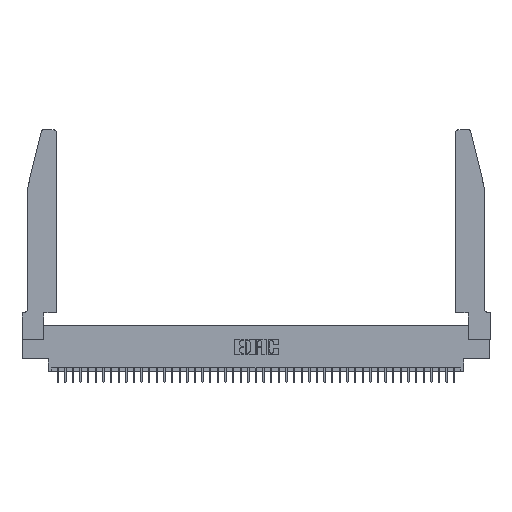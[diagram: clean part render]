
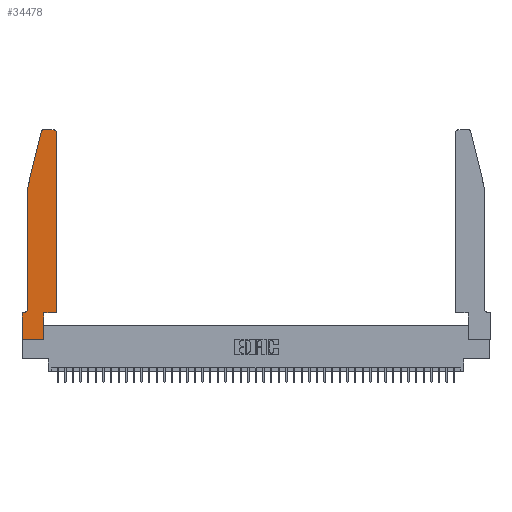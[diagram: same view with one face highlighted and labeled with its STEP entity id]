
A CAD part, top view. The second image highlights one B-rep face of the part: STEP entity #34478.
In plain terms, the highlighted planar face has unit normal (0, 0, 1).
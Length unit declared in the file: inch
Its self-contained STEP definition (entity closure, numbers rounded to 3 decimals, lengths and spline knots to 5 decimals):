
#2469 = ORIENTED_EDGE ( 'NONE', *, *, #20952, .T. ) ;
#2894 = VERTEX_POINT ( 'NONE', #5414 ) ;
#3393 = LINE ( 'NONE', #13477, #7256 ) ;
#3752 = VECTOR ( 'NONE', #13793, 39.37008 ) ;
#3867 = DIRECTION ( 'NONE',  ( -1., 0., 0. ) ) ;
#4237 = ORIENTED_EDGE ( 'NONE', *, *, #17763, .T. ) ;
#4721 = VERTEX_POINT ( 'NONE', #37767 ) ;
#4856 = VERTEX_POINT ( 'NONE', #15403 ) ;
#5414 = CARTESIAN_POINT ( 'NONE',  ( 0.4205, 2.75, 0.37 ) ) ;
#6735 = DIRECTION ( 'NONE',  ( -0.239, -0.971, 0. ) ) ;
#6791 = DIRECTION ( 'NONE',  ( 0., 0., -1. ) ) ;
#6862 = CIRCLE ( 'NONE', #9811, 0.07 ) ;
#7106 = CARTESIAN_POINT ( 'NONE',  ( 0., 0.35, 0.37 ) ) ;
#7256 = VECTOR ( 'NONE', #27380, 39.37008 ) ;
#7772 = ORIENTED_EDGE ( 'NONE', *, *, #38119, .T. ) ;
#7897 = CARTESIAN_POINT ( 'NONE',  ( 0.2865, 0., 0.37 ) ) ;
#8594 = VERTEX_POINT ( 'NONE', #33508 ) ;
#8915 = VERTEX_POINT ( 'NONE', #7897 ) ;
#9157 = ORIENTED_EDGE ( 'NONE', *, *, #35785, .T. ) ;
#9811 = AXIS2_PLACEMENT_3D ( 'NONE', #41248, #6791, #37839 ) ;
#9848 = ORIENTED_EDGE ( 'NONE', *, *, #42678, .T. ) ;
#10182 = ORIENTED_EDGE ( 'NONE', *, *, #14208, .T. ) ;
#10358 = CARTESIAN_POINT ( 'NONE',  ( 0.4505, 0.35, 0.37 ) ) ;
#10992 = VECTOR ( 'NONE', #33091, 39.37008 ) ;
#11718 = EDGE_CURVE ( 'NONE', #22660, #11918, #16778, .T. ) ;
#11918 = VERTEX_POINT ( 'NONE', #24294 ) ;
#13005 = ORIENTED_EDGE ( 'NONE', *, *, #24244, .T. ) ;
#13048 = DIRECTION ( 'NONE',  ( 0., -1., 0. ) ) ;
#13164 = DIRECTION ( 'NONE',  ( 0., 0., 1. ) ) ;
#13477 = CARTESIAN_POINT ( 'NONE',  ( 0., 0., 0.37 ) ) ;
#13793 = DIRECTION ( 'NONE',  ( 0., 1., 0. ) ) ;
#14169 = CARTESIAN_POINT ( 'NONE',  ( 0.2605, 2.75, 0.37 ) ) ;
#14208 = EDGE_CURVE ( 'NONE', #8915, #22660, #39485, .T. ) ;
#14546 = CARTESIAN_POINT ( 'NONE',  ( 0.2865, 0.35, 0.37 ) ) ;
#14649 = FACE_OUTER_BOUND ( 'NONE', #22229, .T. ) ;
#14872 = DIRECTION ( 'NONE',  ( 1., 0., 0. ) ) ;
#15403 = CARTESIAN_POINT ( 'NONE',  ( 0.0755, 0.42, 0.37 ) ) ;
#15844 = AXIS2_PLACEMENT_3D ( 'NONE', #7106, #38838, #14872 ) ;
#16377 = CARTESIAN_POINT ( 'NONE',  ( 0.4205, 2.72, 0.37 ) ) ;
#16703 = LINE ( 'NONE', #20130, #23182 ) ;
#16778 = LINE ( 'NONE', #33859, #42130 ) ;
#16821 = LINE ( 'NONE', #20233, #24595 ) ;
#17763 = EDGE_CURVE ( 'NONE', #8594, #4721, #25350, .T. ) ;
#17779 = EDGE_CURVE ( 'NONE', #2894, #39701, #24451, .T. ) ;
#18990 = CARTESIAN_POINT ( 'NONE',  ( 0.2865, 0.35, 0.37 ) ) ;
#19395 = CARTESIAN_POINT ( 'NONE',  ( 0.0755, 2., 0.37 ) ) ;
#20130 = CARTESIAN_POINT ( 'NONE',  ( 0.0755, 2., 0.37 ) ) ;
#20233 = CARTESIAN_POINT ( 'NONE',  ( 0.0755, 2., 0.37 ) ) ;
#20424 = LINE ( 'NONE', #38190, #29320 ) ;
#20952 = EDGE_CURVE ( 'NONE', #39519, #2894, #44147, .T. ) ;
#22229 = EDGE_LOOP ( 'NONE', ( #31428, #36930, #13005, #9157, #42473, #4237, #7772, #30737, #10182, #41584, #9848, #2469 ) ) ;
#22246 = CARTESIAN_POINT ( 'NONE',  ( 0., 0., 0.37 ) ) ;
#22268 = VECTOR ( 'NONE', #28747, 39.37008 ) ;
#22387 = VERTEX_POINT ( 'NONE', #19395 ) ;
#22660 = VERTEX_POINT ( 'NONE', #14546 ) ;
#23182 = VECTOR ( 'NONE', #13048, 39.37008 ) ;
#24244 = EDGE_CURVE ( 'NONE', #29957, #22387, #16821, .T. ) ;
#24294 = CARTESIAN_POINT ( 'NONE',  ( 0.4505, 0.35, 0.37 ) ) ;
#24451 = LINE ( 'NONE', #14169, #25905 ) ;
#24595 = VECTOR ( 'NONE', #6735, 39.37008 ) ;
#25350 = LINE ( 'NONE', #34931, #22268 ) ;
#25905 = VECTOR ( 'NONE', #3867, 39.37008 ) ;
#25978 = AXIS2_PLACEMENT_3D ( 'NONE', #16377, #40538, #34155 ) ;
#26748 = CARTESIAN_POINT ( 'NONE',  ( 0.25487, 2.72718, 0.37 ) ) ;
#27070 = DIRECTION ( 'NONE',  ( 1., 0., 0. ) ) ;
#27380 = DIRECTION ( 'NONE',  ( 0., -1., 0. ) ) ;
#28747 = DIRECTION ( 'NONE',  ( -1., 0., 0. ) ) ;
#29320 = VECTOR ( 'NONE', #37507, 39.37008 ) ;
#29957 = VERTEX_POINT ( 'NONE', #26748 ) ;
#30478 = CARTESIAN_POINT ( 'NONE',  ( 0.284, 2.72, 0.37 ) ) ;
#30737 = ORIENTED_EDGE ( 'NONE', *, *, #42673, .T. ) ;
#31428 = ORIENTED_EDGE ( 'NONE', *, *, #17779, .T. ) ;
#31615 = EDGE_CURVE ( 'NONE', #4856, #8594, #6862, .T. ) ;
#32009 = AXIS2_PLACEMENT_3D ( 'NONE', #30478, #13164, #27070 ) ;
#33091 = DIRECTION ( 'NONE',  ( 0., 1., 0. ) ) ;
#33508 = CARTESIAN_POINT ( 'NONE',  ( 0.0055, 0.35, 0.37 ) ) ;
#33859 = CARTESIAN_POINT ( 'NONE',  ( 0.4505, 0.35, 0.37 ) ) ;
#34155 = DIRECTION ( 'NONE',  ( 1., 0., 0. ) ) ;
#34174 = CIRCLE ( 'NONE', #32009, 0.03 ) ;
#34478 = ADVANCED_FACE ( 'NONE', ( #14649 ), #38389, .T. ) ;
#34931 = CARTESIAN_POINT ( 'NONE',  ( 0.0755, 0.35, 0.37 ) ) ;
#35785 = EDGE_CURVE ( 'NONE', #22387, #4856, #16703, .T. ) ;
#36031 = CARTESIAN_POINT ( 'NONE',  ( 0.284, 2.75, 0.37 ) ) ;
#36831 = EDGE_CURVE ( 'NONE', #39701, #29957, #34174, .T. ) ;
#36930 = ORIENTED_EDGE ( 'NONE', *, *, #36831, .T. ) ;
#37507 = DIRECTION ( 'NONE',  ( 1., 0., 0. ) ) ;
#37767 = CARTESIAN_POINT ( 'NONE',  ( 0., 0.35, 0.37 ) ) ;
#37839 = DIRECTION ( 'NONE',  ( -1., 0., 0. ) ) ;
#38119 = EDGE_CURVE ( 'NONE', #4721, #38787, #3393, .T. ) ;
#38190 = CARTESIAN_POINT ( 'NONE',  ( 0., 0., 0.37 ) ) ;
#38389 = PLANE ( 'NONE',  #15844 ) ;
#38787 = VERTEX_POINT ( 'NONE', #22246 ) ;
#38838 = DIRECTION ( 'NONE',  ( 0., 0., 1. ) ) ;
#39485 = LINE ( 'NONE', #18990, #10992 ) ;
#39519 = VERTEX_POINT ( 'NONE', #41743 ) ;
#39701 = VERTEX_POINT ( 'NONE', #36031 ) ;
#40538 = DIRECTION ( 'NONE',  ( 0., 0., 1. ) ) ;
#41248 = CARTESIAN_POINT ( 'NONE',  ( 0.0055, 0.42, 0.37 ) ) ;
#41584 = ORIENTED_EDGE ( 'NONE', *, *, #11718, .T. ) ;
#41743 = CARTESIAN_POINT ( 'NONE',  ( 0.4505, 2.72, 0.37 ) ) ;
#42130 = VECTOR ( 'NONE', #43684, 39.37008 ) ;
#42473 = ORIENTED_EDGE ( 'NONE', *, *, #31615, .T. ) ;
#42673 = EDGE_CURVE ( 'NONE', #38787, #8915, #20424, .T. ) ;
#42678 = EDGE_CURVE ( 'NONE', #11918, #39519, #44345, .T. ) ;
#43684 = DIRECTION ( 'NONE',  ( 1., 0., 0. ) ) ;
#44147 = CIRCLE ( 'NONE', #25978, 0.03 ) ;
#44345 = LINE ( 'NONE', #10358, #3752 ) ;
